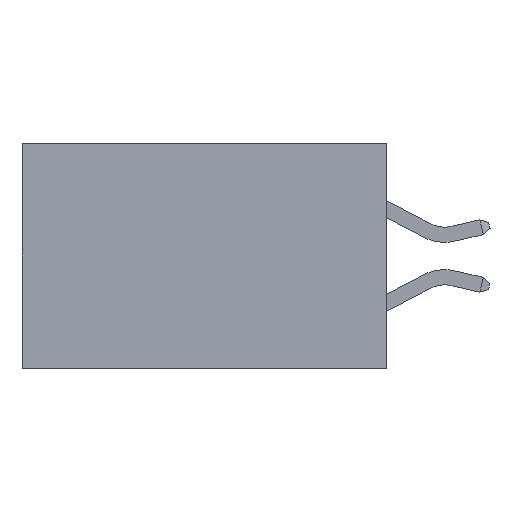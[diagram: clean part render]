
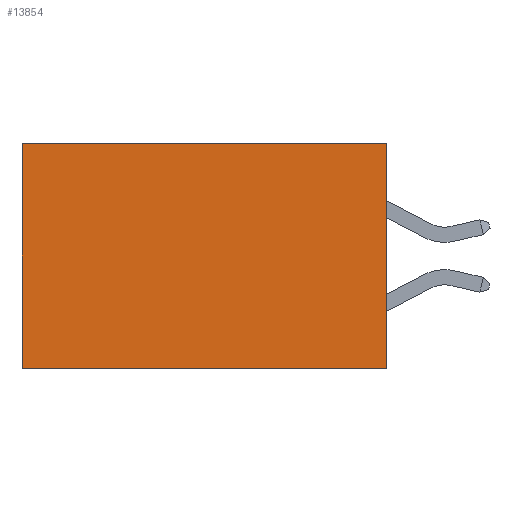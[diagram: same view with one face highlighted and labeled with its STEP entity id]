
A CAD part, left-side view. The second image highlights one B-rep face of the part: STEP entity #13854.
In plain terms, the highlighted planar face has unit normal (-1, 0, 0).
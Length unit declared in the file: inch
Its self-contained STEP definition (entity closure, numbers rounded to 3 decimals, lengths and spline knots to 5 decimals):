
#144 = DIRECTION ( 'NONE',  ( 0., 0., -1. ) ) ;
#648 = CARTESIAN_POINT ( 'NONE',  ( 0.298, 0.6, -0.37 ) ) ;
#1243 = VERTEX_POINT ( 'NONE', #1555 ) ;
#1365 = VECTOR ( 'NONE', #4538, 39.37008 ) ;
#1555 = CARTESIAN_POINT ( 'NONE',  ( 0.298, 0., 0. ) ) ;
#1904 = ORIENTED_EDGE ( 'NONE', *, *, #11443, .F. ) ;
#2534 = DIRECTION ( 'NONE',  ( 0., 1., 0. ) ) ;
#2695 = ORIENTED_EDGE ( 'NONE', *, *, #9845, .F. ) ;
#3051 = EDGE_LOOP ( 'NONE', ( #8454, #1904, #2695, #11985 ) ) ;
#3917 = VERTEX_POINT ( 'NONE', #11234 ) ;
#4148 = VERTEX_POINT ( 'NONE', #648 ) ;
#4356 = LINE ( 'NONE', #11731, #1365 ) ;
#4538 = DIRECTION ( 'NONE',  ( 0., 0., -1. ) ) ;
#5187 = CARTESIAN_POINT ( 'NONE',  ( 0.298, 0., 0. ) ) ;
#5205 = LINE ( 'NONE', #11046, #14416 ) ;
#6471 = PLANE ( 'NONE',  #8126 ) ;
#7117 = VECTOR ( 'NONE', #12854, 39.37008 ) ;
#7228 = CARTESIAN_POINT ( 'NONE',  ( 0.298, 0.6, 0. ) ) ;
#7711 = DIRECTION ( 'NONE',  ( 1., 0., 0. ) ) ;
#7995 = LINE ( 'NONE', #12264, #13910 ) ;
#8126 = AXIS2_PLACEMENT_3D ( 'NONE', #5187, #7711, #144 ) ;
#8454 = ORIENTED_EDGE ( 'NONE', *, *, #8803, .T. ) ;
#8803 = EDGE_CURVE ( 'NONE', #10386, #4148, #4356, .T. ) ;
#9764 = FACE_OUTER_BOUND ( 'NONE', #3051, .T. ) ;
#9845 = EDGE_CURVE ( 'NONE', #1243, #3917, #10604, .T. ) ;
#10386 = VERTEX_POINT ( 'NONE', #7228 ) ;
#10604 = LINE ( 'NONE', #11643, #7117 ) ;
#11046 = CARTESIAN_POINT ( 'NONE',  ( 0.298, 0., 0. ) ) ;
#11234 = CARTESIAN_POINT ( 'NONE',  ( 0.298, 0., -0.37 ) ) ;
#11443 = EDGE_CURVE ( 'NONE', #3917, #4148, #7995, .T. ) ;
#11643 = CARTESIAN_POINT ( 'NONE',  ( 0.298, 0., 0. ) ) ;
#11731 = CARTESIAN_POINT ( 'NONE',  ( 0.298, 0.6, 0. ) ) ;
#11985 = ORIENTED_EDGE ( 'NONE', *, *, #14202, .T. ) ;
#12264 = CARTESIAN_POINT ( 'NONE',  ( 0.298, 0., -0.37 ) ) ;
#12854 = DIRECTION ( 'NONE',  ( 0., 0., -1. ) ) ;
#13854 = ADVANCED_FACE ( 'NONE', ( #9764 ), #6471, .F. ) ;
#13910 = VECTOR ( 'NONE', #14704, 39.37008 ) ;
#14202 = EDGE_CURVE ( 'NONE', #1243, #10386, #5205, .T. ) ;
#14416 = VECTOR ( 'NONE', #2534, 39.37008 ) ;
#14704 = DIRECTION ( 'NONE',  ( 0., 1., 0. ) ) ;
